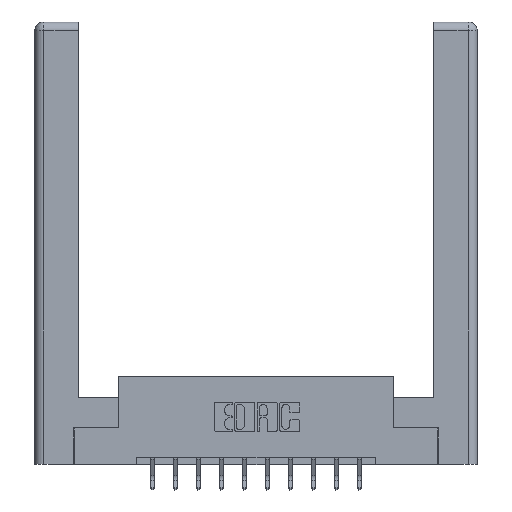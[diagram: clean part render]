
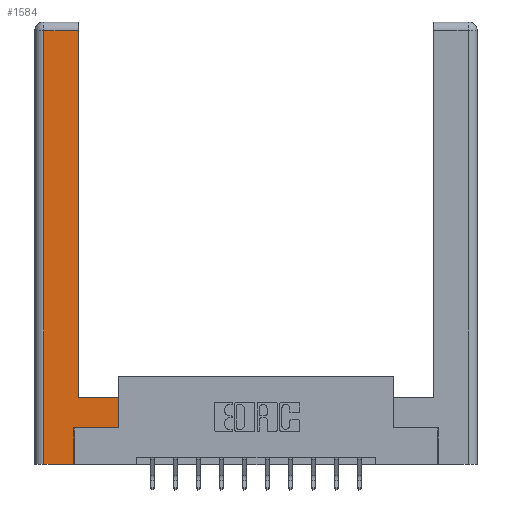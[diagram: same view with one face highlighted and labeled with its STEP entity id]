
A CAD part, top view. The second image highlights one B-rep face of the part: STEP entity #1584.
In plain terms, the highlighted planar face has unit normal (0, 0, 1).
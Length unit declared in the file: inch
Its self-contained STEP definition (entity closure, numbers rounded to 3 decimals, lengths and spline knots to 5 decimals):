
#872 = VECTOR ( 'NONE', #6120, 39.37008 ) ;
#885 = DIRECTION ( 'NONE',  ( 0., 0., -1. ) ) ;
#889 = EDGE_CURVE ( 'NONE', #13484, #9288, #13747, .T. ) ;
#904 = VECTOR ( 'NONE', #14187, 39.37008 ) ;
#1306 = LINE ( 'NONE', #13254, #1483 ) ;
#1451 = CARTESIAN_POINT ( 'NONE',  ( 0.0615, 0., 0. ) ) ;
#1483 = VECTOR ( 'NONE', #6418, 39.37008 ) ;
#1584 = ADVANCED_FACE ( 'NONE', ( #11249 ), #7739, .F. ) ;
#1738 = DIRECTION ( 'NONE',  ( 1., 0., 0. ) ) ;
#1796 = EDGE_CURVE ( 'NONE', #9288, #1862, #11409, .T. ) ;
#1862 = VERTEX_POINT ( 'NONE', #8239 ) ;
#2088 = EDGE_CURVE ( 'NONE', #3189, #10568, #4623, .T. ) ;
#2102 = CARTESIAN_POINT ( 'NONE',  ( 0.295, 0.45, 0. ) ) ;
#2218 = ORIENTED_EDGE ( 'NONE', *, *, #14275, .T. ) ;
#2280 = CARTESIAN_POINT ( 'NONE',  ( 0.565, 0.245, 0. ) ) ;
#2673 = EDGE_LOOP ( 'NONE', ( #5579, #10824, #2218, #2968, #4510, #14269, #3567, #9758 ) ) ;
#2706 = VERTEX_POINT ( 'NONE', #7319 ) ;
#2882 = CARTESIAN_POINT ( 'NONE',  ( 0.265, 0., 0. ) ) ;
#2968 = ORIENTED_EDGE ( 'NONE', *, *, #2088, .T. ) ;
#3189 = VERTEX_POINT ( 'NONE', #1451 ) ;
#3259 = CARTESIAN_POINT ( 'NONE',  ( 0.0615, 2.94, 0. ) ) ;
#3268 = CARTESIAN_POINT ( 'NONE',  ( 0.295, 0.45, 0. ) ) ;
#3567 = ORIENTED_EDGE ( 'NONE', *, *, #1796, .T. ) ;
#3574 = LINE ( 'NONE', #3268, #13774 ) ;
#4144 = EDGE_CURVE ( 'NONE', #13430, #10767, #5293, .T. ) ;
#4243 = DIRECTION ( 'NONE',  ( 0., 1., 0. ) ) ;
#4510 = ORIENTED_EDGE ( 'NONE', *, *, #7579, .T. ) ;
#4623 = LINE ( 'NONE', #2882, #13391 ) ;
#4871 = EDGE_CURVE ( 'NONE', #10767, #2706, #10451, .T. ) ;
#4998 = CARTESIAN_POINT ( 'NONE',  ( 0.0615, 0., 0. ) ) ;
#5293 = LINE ( 'NONE', #13323, #12423 ) ;
#5399 = CARTESIAN_POINT ( 'NONE',  ( 0.295, 2.94, 0. ) ) ;
#5579 = ORIENTED_EDGE ( 'NONE', *, *, #4144, .T. ) ;
#6120 = DIRECTION ( 'NONE',  ( 0., 1., 0. ) ) ;
#6418 = DIRECTION ( 'NONE',  ( 0., 1., 0. ) ) ;
#6551 = EDGE_CURVE ( 'NONE', #1862, #13430, #3574, .T. ) ;
#6990 = CARTESIAN_POINT ( 'NONE',  ( 0.265, 0.245, 0. ) ) ;
#7319 = CARTESIAN_POINT ( 'NONE',  ( 0.0615, 2.94, 0. ) ) ;
#7579 = EDGE_CURVE ( 'NONE', #10568, #13484, #1306, .T. ) ;
#7739 = PLANE ( 'NONE',  #12247 ) ;
#8031 = VECTOR ( 'NONE', #10500, 39.37008 ) ;
#8239 = CARTESIAN_POINT ( 'NONE',  ( 0.565, 0.45, 0. ) ) ;
#8287 = CARTESIAN_POINT ( 'NONE',  ( 0.565, 0.45, 0. ) ) ;
#8857 = DIRECTION ( 'NONE',  ( -1., 0., 0. ) ) ;
#9279 = CARTESIAN_POINT ( 'NONE',  ( 0.565, 0.245, 0. ) ) ;
#9288 = VERTEX_POINT ( 'NONE', #2280 ) ;
#9330 = CARTESIAN_POINT ( 'NONE',  ( 0.265, 0., 0. ) ) ;
#9758 = ORIENTED_EDGE ( 'NONE', *, *, #6551, .T. ) ;
#10175 = DIRECTION ( 'NONE',  ( -1., 0., 0. ) ) ;
#10451 = LINE ( 'NONE', #3259, #11174 ) ;
#10500 = DIRECTION ( 'NONE',  ( 1., 0., 0. ) ) ;
#10568 = VERTEX_POINT ( 'NONE', #9330 ) ;
#10767 = VERTEX_POINT ( 'NONE', #5399 ) ;
#10824 = ORIENTED_EDGE ( 'NONE', *, *, #4871, .T. ) ;
#11174 = VECTOR ( 'NONE', #8857, 39.37008 ) ;
#11186 = DIRECTION ( 'NONE',  ( -1., 0., 0. ) ) ;
#11249 = FACE_OUTER_BOUND ( 'NONE', #2673, .T. ) ;
#11409 = LINE ( 'NONE', #8287, #872 ) ;
#12247 = AXIS2_PLACEMENT_3D ( 'NONE', #13286, #885, #11186 ) ;
#12423 = VECTOR ( 'NONE', #4243, 39.37008 ) ;
#13254 = CARTESIAN_POINT ( 'NONE',  ( 0.265, 0.245, 0. ) ) ;
#13286 = CARTESIAN_POINT ( 'NONE',  ( 0., 0., 0. ) ) ;
#13323 = CARTESIAN_POINT ( 'NONE',  ( 0.295, 3., 0. ) ) ;
#13391 = VECTOR ( 'NONE', #1738, 39.37008 ) ;
#13430 = VERTEX_POINT ( 'NONE', #2102 ) ;
#13484 = VERTEX_POINT ( 'NONE', #6990 ) ;
#13747 = LINE ( 'NONE', #9279, #8031 ) ;
#13774 = VECTOR ( 'NONE', #10175, 39.37008 ) ;
#14187 = DIRECTION ( 'NONE',  ( 0., -1., 0. ) ) ;
#14269 = ORIENTED_EDGE ( 'NONE', *, *, #889, .T. ) ;
#14275 = EDGE_CURVE ( 'NONE', #2706, #3189, #14302, .T. ) ;
#14302 = LINE ( 'NONE', #4998, #904 ) ;
